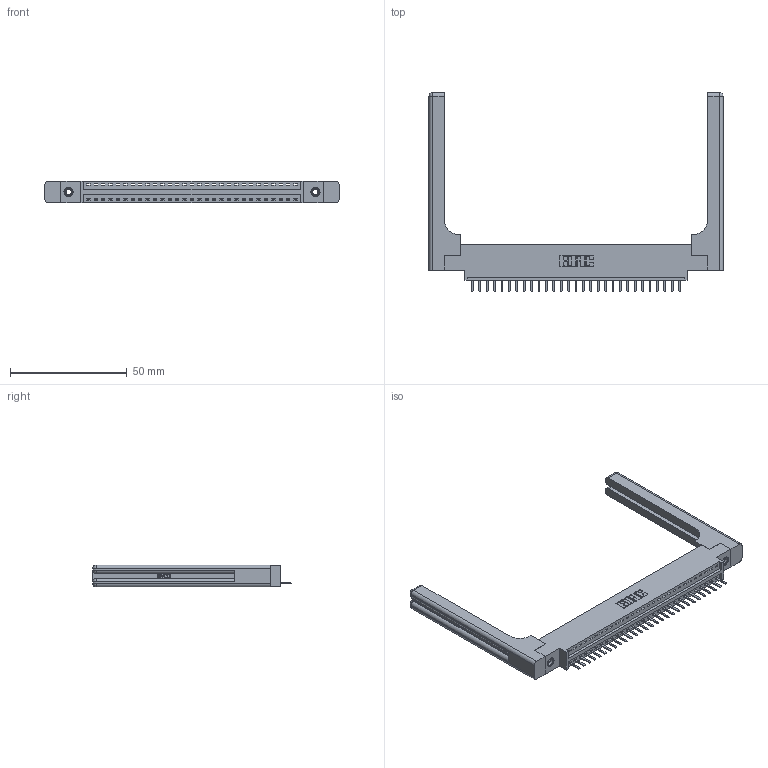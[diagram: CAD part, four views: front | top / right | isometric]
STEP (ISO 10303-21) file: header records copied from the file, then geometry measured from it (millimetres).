
FILE_DESCRIPTION (( 'STEP AP203' ), '1' );
FILE_NAME ('346-029-520-658.STEP', '2022-05-06T08:33:28', ( '' ), ( '' ), 'SwSTEP 2.0', 'SolidWorks 2020', '' );
FILE_SCHEMA (( 'CONFIG_CONTROL_DESIGN' ));
Length unit declared in the file: inch
Products named in the file (5): 345-292-001_345-293-120; 346-220-058_345-220-058; 346-029-520-658; 345-250-001_345-250-001-102; 346 Part_0.170 Offset - 0.156 Dia-TH
Assembly tree (34 placements, depth 2):
  346-029-520-658
    346 Part_0.170 Offset - 0.156 Dia-TH
    345-292-001_345-293-120  x29
    345-250-001_345-250-001-102  x2
    346-220-058_345-220-058  x2
Bounding box: 126.14 x 85.29 x 9.4 mm (x, y, z)
Volume: 19246.7 mm3; surface area: 19602.3 mm2
Topology: 34 solids, 34 shells, 2194 faces, 6379 edges, 4154 vertices
Faces by surface type: plane 1460, cylinder 674, bspline 36, cone 12, sphere 8, torus 4
Entity records: 25592 total; most frequent: CARTESIAN_POINT 5386, ORIENTED_EDGE 4132, DIRECTION 3684, EDGE_CURVE 2066, VECTOR 1722, LINE 1722, VERTEX_POINT 1366, AXIS2_PLACEMENT_3D 981
